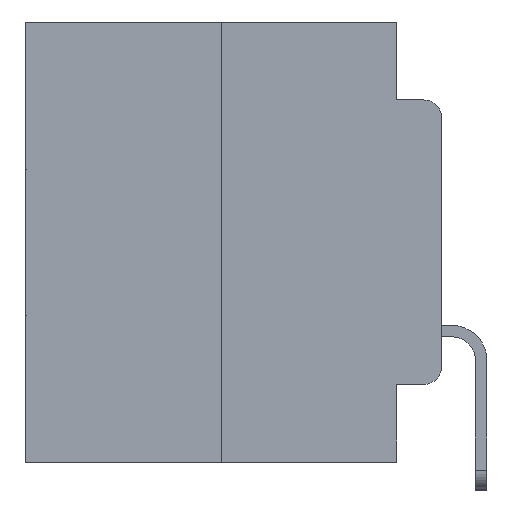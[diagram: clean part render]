
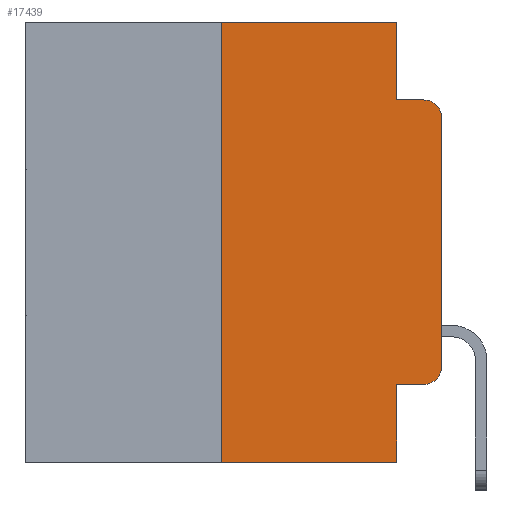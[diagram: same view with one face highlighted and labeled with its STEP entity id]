
A CAD part, left-side view. The second image highlights one B-rep face of the part: STEP entity #17439.
In plain terms, the highlighted planar face has unit normal (-1, 0, 0).
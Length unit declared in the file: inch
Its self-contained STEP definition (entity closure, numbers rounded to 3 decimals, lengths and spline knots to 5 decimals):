
#179 = EDGE_CURVE ( 'NONE', #23950, #2509, #15407, .T. ) ;
#309 = CARTESIAN_POINT ( 'NONE',  ( 0., 0.25, 0. ) ) ;
#806 = VERTEX_POINT ( 'NONE', #14388 ) ;
#2233 = AXIS2_PLACEMENT_3D ( 'NONE', #11013, #13285, #27992 ) ;
#2354 = VERTEX_POINT ( 'NONE', #309 ) ;
#2509 = VERTEX_POINT ( 'NONE', #5195 ) ;
#3542 = VECTOR ( 'NONE', #21241, 39.37008 ) ;
#4289 = LINE ( 'NONE', #19115, #3542 ) ;
#4391 = VECTOR ( 'NONE', #14133, 39.37008 ) ;
#5143 = LINE ( 'NONE', #11863, #4391 ) ;
#5195 = CARTESIAN_POINT ( 'NONE',  ( 0., 0.02, -0.0885 ) ) ;
#5320 = VECTOR ( 'NONE', #20085, 39.37008 ) ;
#5333 = CARTESIAN_POINT ( 'NONE',  ( 0., 0.051, -0.0885 ) ) ;
#5808 = CARTESIAN_POINT ( 'NONE',  ( 0., 0.02, -0.1085 ) ) ;
#5879 = DIRECTION ( 'NONE',  ( 0., -1., 0. ) ) ;
#6578 = CARTESIAN_POINT ( 'NONE',  ( 0., 0.051, -0.4115 ) ) ;
#7176 = CARTESIAN_POINT ( 'NONE',  ( 0., 0.02, -0.4115 ) ) ;
#7231 = EDGE_CURVE ( 'NONE', #12126, #2354, #17257, .T. ) ;
#7250 = DIRECTION ( 'NONE',  ( -1., 0., 0. ) ) ;
#7469 = ORIENTED_EDGE ( 'NONE', *, *, #12262, .F. ) ;
#7717 = EDGE_LOOP ( 'NONE', ( #16643, #27408, #25211, #13496, #7469, #21279, #24585, #28372, #19647, #17097 ) ) ;
#8156 = DIRECTION ( 'NONE',  ( 0., 0., -1. ) ) ;
#8724 = AXIS2_PLACEMENT_3D ( 'NONE', #5808, #21301, #8156 ) ;
#8931 = VECTOR ( 'NONE', #11210, 39.37008 ) ;
#10207 = CIRCLE ( 'NONE', #8724, 0.02 ) ;
#10467 = DIRECTION ( 'NONE',  ( 0., -1., 0. ) ) ;
#10550 = VERTEX_POINT ( 'NONE', #10980 ) ;
#10980 = CARTESIAN_POINT ( 'NONE',  ( 0., 0.051, -0.4115 ) ) ;
#11013 = CARTESIAN_POINT ( 'NONE',  ( 0., 0.473, 0. ) ) ;
#11165 = CARTESIAN_POINT ( 'NONE',  ( 0., 0.051, 0. ) ) ;
#11210 = DIRECTION ( 'NONE',  ( 0., -1., 0. ) ) ;
#11221 = FACE_OUTER_BOUND ( 'NONE', #7717, .T. ) ;
#11551 = VECTOR ( 'NONE', #5879, 39.37008 ) ;
#11863 = CARTESIAN_POINT ( 'NONE',  ( 0., 0., 0. ) ) ;
#12126 = VERTEX_POINT ( 'NONE', #19617 ) ;
#12262 = EDGE_CURVE ( 'NONE', #2354, #806, #27713, .T. ) ;
#12886 = LINE ( 'NONE', #11165, #13596 ) ;
#12963 = LINE ( 'NONE', #19228, #11551 ) ;
#13285 = DIRECTION ( 'NONE',  ( 1., 0., 0. ) ) ;
#13434 = DIRECTION ( 'NONE',  ( 0., 0., -1. ) ) ;
#13496 = ORIENTED_EDGE ( 'NONE', *, *, #24085, .F. ) ;
#13596 = VECTOR ( 'NONE', #13434, 39.37008 ) ;
#13891 = CARTESIAN_POINT ( 'NONE',  ( 0., 0.25, 0. ) ) ;
#14133 = DIRECTION ( 'NONE',  ( 0., 0., 1. ) ) ;
#14388 = CARTESIAN_POINT ( 'NONE',  ( 0., 0.051, 0. ) ) ;
#14731 = VECTOR ( 'NONE', #10467, 39.37008 ) ;
#14900 = LINE ( 'NONE', #6578, #8931 ) ;
#15347 = VERTEX_POINT ( 'NONE', #19110 ) ;
#15407 = LINE ( 'NONE', #16872, #14731 ) ;
#16643 = ORIENTED_EDGE ( 'NONE', *, *, #18370, .T. ) ;
#16795 = CARTESIAN_POINT ( 'NONE',  ( 0., 0., -0.1085 ) ) ;
#16872 = CARTESIAN_POINT ( 'NONE',  ( 0., 0.051, -0.0885 ) ) ;
#16919 = EDGE_CURVE ( 'NONE', #18576, #2509, #10207, .T. ) ;
#17097 = ORIENTED_EDGE ( 'NONE', *, *, #24616, .T. ) ;
#17257 = LINE ( 'NONE', #13891, #24156 ) ;
#17439 = ADVANCED_FACE ( 'NONE', ( #11221 ), #23941, .F. ) ;
#18370 = EDGE_CURVE ( 'NONE', #28097, #18576, #5143, .T. ) ;
#18576 = VERTEX_POINT ( 'NONE', #16795 ) ;
#19110 = CARTESIAN_POINT ( 'NONE',  ( 0., 0.051, -0.5 ) ) ;
#19115 = CARTESIAN_POINT ( 'NONE',  ( 0., 0.051, 0. ) ) ;
#19228 = CARTESIAN_POINT ( 'NONE',  ( 0., 0.473, -0.5 ) ) ;
#19617 = CARTESIAN_POINT ( 'NONE',  ( 0., 0.25, -0.5 ) ) ;
#19647 = ORIENTED_EDGE ( 'NONE', *, *, #27330, .T. ) ;
#19654 = EDGE_CURVE ( 'NONE', #12126, #15347, #12963, .T. ) ;
#20085 = DIRECTION ( 'NONE',  ( 0., -1., 0. ) ) ;
#20095 = DIRECTION ( 'NONE',  ( 0., 0., 1. ) ) ;
#20487 = CARTESIAN_POINT ( 'NONE',  ( 0., 0.02, -0.3915 ) ) ;
#20674 = CIRCLE ( 'NONE', #26829, 0.02 ) ;
#21241 = DIRECTION ( 'NONE',  ( 0., 0., -1. ) ) ;
#21279 = ORIENTED_EDGE ( 'NONE', *, *, #7231, .F. ) ;
#21301 = DIRECTION ( 'NONE',  ( -1., 0., 0. ) ) ;
#22611 = DIRECTION ( 'NONE',  ( 0., 0., -1. ) ) ;
#22638 = VERTEX_POINT ( 'NONE', #7176 ) ;
#23922 = CARTESIAN_POINT ( 'NONE',  ( 0., 0., -0.3915 ) ) ;
#23941 = PLANE ( 'NONE',  #2233 ) ;
#23950 = VERTEX_POINT ( 'NONE', #5333 ) ;
#24085 = EDGE_CURVE ( 'NONE', #806, #23950, #4289, .T. ) ;
#24156 = VECTOR ( 'NONE', #20095, 39.37008 ) ;
#24299 = CARTESIAN_POINT ( 'NONE',  ( 0., 0.473, 0. ) ) ;
#24585 = ORIENTED_EDGE ( 'NONE', *, *, #19654, .T. ) ;
#24616 = EDGE_CURVE ( 'NONE', #22638, #28097, #20674, .T. ) ;
#24714 = EDGE_CURVE ( 'NONE', #10550, #15347, #12886, .T. ) ;
#25211 = ORIENTED_EDGE ( 'NONE', *, *, #179, .F. ) ;
#26829 = AXIS2_PLACEMENT_3D ( 'NONE', #20487, #7250, #22611 ) ;
#27330 = EDGE_CURVE ( 'NONE', #10550, #22638, #14900, .T. ) ;
#27408 = ORIENTED_EDGE ( 'NONE', *, *, #16919, .T. ) ;
#27713 = LINE ( 'NONE', #24299, #5320 ) ;
#27992 = DIRECTION ( 'NONE',  ( 0., 0., -1. ) ) ;
#28097 = VERTEX_POINT ( 'NONE', #23922 ) ;
#28372 = ORIENTED_EDGE ( 'NONE', *, *, #24714, .F. ) ;
